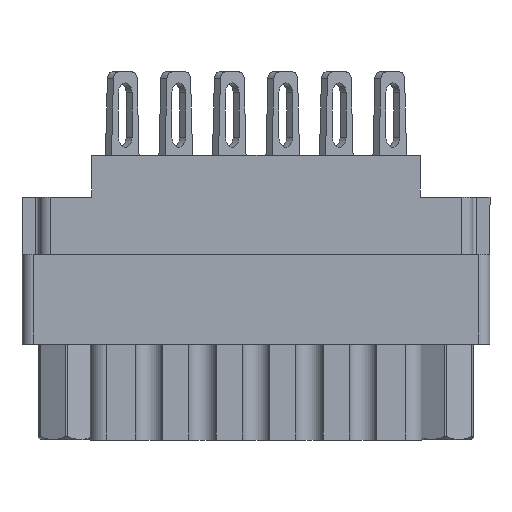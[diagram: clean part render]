
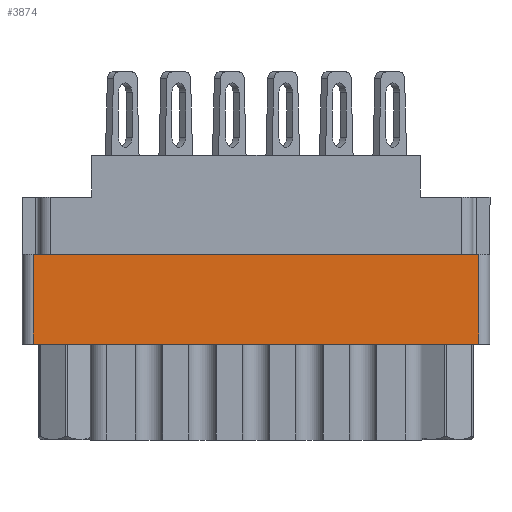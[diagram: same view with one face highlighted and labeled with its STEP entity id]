
A CAD part, front view. The second image highlights one B-rep face of the part: STEP entity #3874.
In plain terms, the highlighted planar face has unit normal (0, -1, 0).
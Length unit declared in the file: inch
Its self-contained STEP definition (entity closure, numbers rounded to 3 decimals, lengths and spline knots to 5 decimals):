
#329 = VERTEX_POINT ( 'NONE', #27117 ) ;
#392 = ORIENTED_EDGE ( 'NONE', *, *, #26141, .F. ) ;
#791 = CARTESIAN_POINT ( 'NONE',  ( 0.624, -0.343, -0.529 ) ) ;
#1127 = CARTESIAN_POINT ( 'NONE',  ( -0.624, -0.343, -0.277 ) ) ;
#1273 = DIRECTION ( 'NONE',  ( 1., 0., 0. ) ) ;
#1823 = VERTEX_POINT ( 'NONE', #791 ) ;
#1901 = VERTEX_POINT ( 'NONE', #1127 ) ;
#2881 = VECTOR ( 'NONE', #1273, 39.37008 ) ;
#3577 = CARTESIAN_POINT ( 'NONE',  ( -0.656, -0.343, -0.277 ) ) ;
#3649 = VECTOR ( 'NONE', #30521, 39.37008 ) ;
#3874 = ADVANCED_FACE ( 'NONE', ( #4388 ), #24508, .T. ) ;
#4388 = FACE_OUTER_BOUND ( 'NONE', #29057, .T. ) ;
#5306 = LINE ( 'NONE', #25436, #19608 ) ;
#8683 = DIRECTION ( 'NONE',  ( 0., -1., 0. ) ) ;
#10120 = CARTESIAN_POINT ( 'NONE',  ( -0.624, -0.343, -0.798 ) ) ;
#11447 = EDGE_CURVE ( 'NONE', #1901, #329, #16119, .T. ) ;
#12269 = ORIENTED_EDGE ( 'NONE', *, *, #18216, .F. ) ;
#13526 = CARTESIAN_POINT ( 'NONE',  ( 0.624, -0.343, -0.798 ) ) ;
#15531 = DIRECTION ( 'NONE',  ( -1., 0., 0. ) ) ;
#16119 = LINE ( 'NONE', #3577, #2881 ) ;
#18216 = EDGE_CURVE ( 'NONE', #25343, #1901, #22648, .T. ) ;
#19087 = DIRECTION ( 'NONE',  ( 0., 0., 1. ) ) ;
#19608 = VECTOR ( 'NONE', #15531, 39.37008 ) ;
#22648 = LINE ( 'NONE', #10120, #29974 ) ;
#22682 = AXIS2_PLACEMENT_3D ( 'NONE', #31290, #8683, #24165 ) ;
#22940 = ORIENTED_EDGE ( 'NONE', *, *, #31759, .T. ) ;
#23090 = LINE ( 'NONE', #13526, #3649 ) ;
#23426 = ORIENTED_EDGE ( 'NONE', *, *, #11447, .F. ) ;
#24165 = DIRECTION ( 'NONE',  ( 0., 0., -1. ) ) ;
#24508 = PLANE ( 'NONE',  #22682 ) ;
#25343 = VERTEX_POINT ( 'NONE', #27321 ) ;
#25436 = CARTESIAN_POINT ( 'NONE',  ( 0.624, -0.343, -0.529 ) ) ;
#26141 = EDGE_CURVE ( 'NONE', #1823, #25343, #5306, .T. ) ;
#27117 = CARTESIAN_POINT ( 'NONE',  ( 0.624, -0.343, -0.277 ) ) ;
#27321 = CARTESIAN_POINT ( 'NONE',  ( -0.624, -0.343, -0.529 ) ) ;
#29057 = EDGE_LOOP ( 'NONE', ( #12269, #392, #22940, #23426 ) ) ;
#29974 = VECTOR ( 'NONE', #19087, 39.37008 ) ;
#30521 = DIRECTION ( 'NONE',  ( 0., 0., 1. ) ) ;
#31290 = CARTESIAN_POINT ( 'NONE',  ( -0.624, -0.343, -0.798 ) ) ;
#31759 = EDGE_CURVE ( 'NONE', #1823, #329, #23090, .T. ) ;
